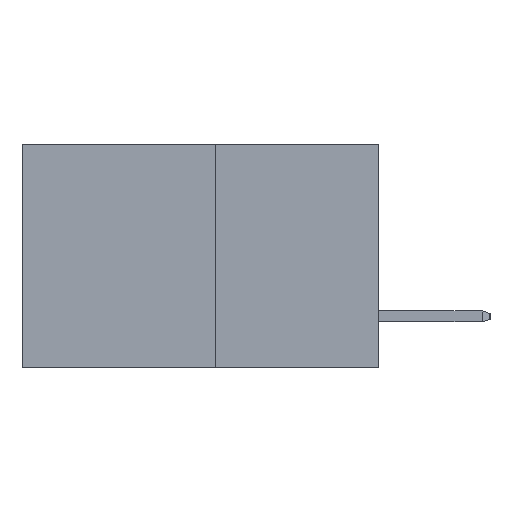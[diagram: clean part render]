
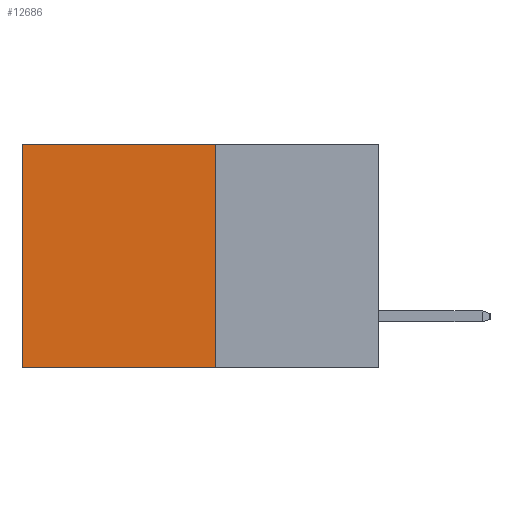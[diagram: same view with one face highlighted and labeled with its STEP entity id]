
A CAD part, left-side view. The second image highlights one B-rep face of the part: STEP entity #12686.
In plain terms, the highlighted planar face has unit normal (-1, 0, 0).
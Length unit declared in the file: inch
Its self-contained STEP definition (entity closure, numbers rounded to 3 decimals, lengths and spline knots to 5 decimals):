
#789 = PLANE ( 'NONE',  #13598 ) ;
#2355 = DIRECTION ( 'NONE',  ( 0., 0., -1. ) ) ;
#2727 = VERTEX_POINT ( 'NONE', #17810 ) ;
#3125 = EDGE_CURVE ( 'NONE', #4552, #17277, #17144, .T. ) ;
#3476 = CARTESIAN_POINT ( 'NONE',  ( 0.277, 0.27, 0. ) ) ;
#3522 = ORIENTED_EDGE ( 'NONE', *, *, #3609, .F. ) ;
#3609 = EDGE_CURVE ( 'NONE', #17277, #4344, #17515, .T. ) ;
#4344 = VERTEX_POINT ( 'NONE', #5028 ) ;
#4543 = CARTESIAN_POINT ( 'NONE',  ( 0.277, 0.59, -0.37 ) ) ;
#4552 = VERTEX_POINT ( 'NONE', #3476 ) ;
#4992 = ORIENTED_EDGE ( 'NONE', *, *, #12424, .T. ) ;
#5028 = CARTESIAN_POINT ( 'NONE',  ( 0.277, 0.59, -0.37 ) ) ;
#5040 = VECTOR ( 'NONE', #6260, 39.37008 ) ;
#5499 = LINE ( 'NONE', #4543, #5040 ) ;
#6260 = DIRECTION ( 'NONE',  ( 0., 0., -1. ) ) ;
#7214 = EDGE_LOOP ( 'NONE', ( #4992, #3522, #14731, #8051 ) ) ;
#7704 = FACE_OUTER_BOUND ( 'NONE', #7214, .T. ) ;
#8051 = ORIENTED_EDGE ( 'NONE', *, *, #8889, .T. ) ;
#8518 = LINE ( 'NONE', #15184, #15177 ) ;
#8889 = EDGE_CURVE ( 'NONE', #4552, #2727, #8518, .T. ) ;
#10616 = DIRECTION ( 'NONE',  ( 0., 1., 0. ) ) ;
#10697 = CARTESIAN_POINT ( 'NONE',  ( 0.277, 0.27, -0.37 ) ) ;
#11086 = DIRECTION ( 'NONE',  ( 1., 0., 0. ) ) ;
#12032 = CARTESIAN_POINT ( 'NONE',  ( 0.277, 0.27, -0.37 ) ) ;
#12362 = CARTESIAN_POINT ( 'NONE',  ( 0.277, 0.27, -0.37 ) ) ;
#12424 = EDGE_CURVE ( 'NONE', #2727, #4344, #5499, .T. ) ;
#12686 = ADVANCED_FACE ( 'NONE', ( #7704 ), #789, .F. ) ;
#13598 = AXIS2_PLACEMENT_3D ( 'NONE', #12362, #11086, #2355 ) ;
#13850 = VECTOR ( 'NONE', #10616, 39.37008 ) ;
#14326 = DIRECTION ( 'NONE',  ( 0., 0., -1. ) ) ;
#14344 = CARTESIAN_POINT ( 'NONE',  ( 0.277, 0.27, -0.37 ) ) ;
#14731 = ORIENTED_EDGE ( 'NONE', *, *, #3125, .F. ) ;
#15177 = VECTOR ( 'NONE', #16555, 39.37008 ) ;
#15184 = CARTESIAN_POINT ( 'NONE',  ( 0.277, 0.27, 0. ) ) ;
#16555 = DIRECTION ( 'NONE',  ( 0., 1., 0. ) ) ;
#16721 = VECTOR ( 'NONE', #14326, 39.37008 ) ;
#17144 = LINE ( 'NONE', #14344, #16721 ) ;
#17277 = VERTEX_POINT ( 'NONE', #12032 ) ;
#17515 = LINE ( 'NONE', #10697, #13850 ) ;
#17810 = CARTESIAN_POINT ( 'NONE',  ( 0.277, 0.59, 0. ) ) ;
